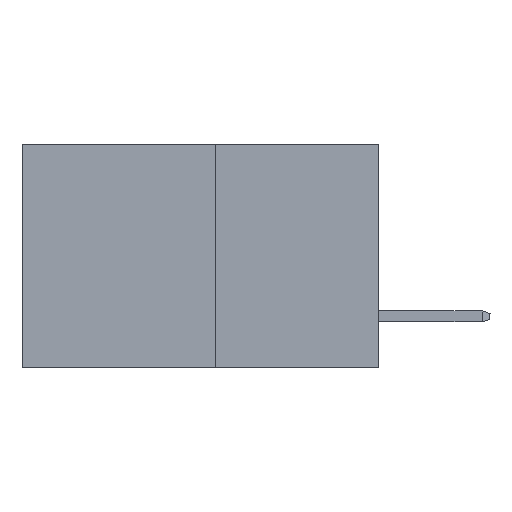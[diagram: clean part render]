
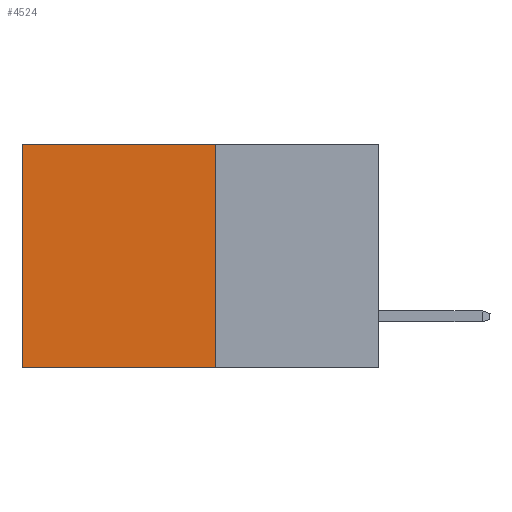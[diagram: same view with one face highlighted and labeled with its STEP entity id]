
A CAD part, left-side view. The second image highlights one B-rep face of the part: STEP entity #4524.
In plain terms, the highlighted planar face has unit normal (-1, 0, 0).
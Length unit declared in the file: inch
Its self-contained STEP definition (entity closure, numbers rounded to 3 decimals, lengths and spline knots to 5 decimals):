
#132 = VECTOR ( 'NONE', #27790, 39.37008 ) ;
#869 = LINE ( 'NONE', #1344, #132 ) ;
#1261 = CARTESIAN_POINT ( 'NONE',  ( 0.277, 0.59, 0. ) ) ;
#1344 = CARTESIAN_POINT ( 'NONE',  ( 0.277, 0.27, -0.37 ) ) ;
#2692 = DIRECTION ( 'NONE',  ( 0., 0., -1. ) ) ;
#3535 = ORIENTED_EDGE ( 'NONE', *, *, #17975, .T. ) ;
#4341 = CARTESIAN_POINT ( 'NONE',  ( 0.277, 0.27, -0.37 ) ) ;
#4524 = ADVANCED_FACE ( 'NONE', ( #17333 ), #16282, .F. ) ;
#4941 = EDGE_CURVE ( 'NONE', #23599, #19851, #16591, .T. ) ;
#6849 = CARTESIAN_POINT ( 'NONE',  ( 0.277, 0.59, -0.37 ) ) ;
#7403 = VECTOR ( 'NONE', #23509, 39.37008 ) ;
#7440 = VERTEX_POINT ( 'NONE', #21478 ) ;
#8963 = CARTESIAN_POINT ( 'NONE',  ( 0.277, 0.27, -0.37 ) ) ;
#9587 = AXIS2_PLACEMENT_3D ( 'NONE', #17483, #15407, #20422 ) ;
#10596 = ORIENTED_EDGE ( 'NONE', *, *, #11051, .F. ) ;
#10961 = ORIENTED_EDGE ( 'NONE', *, *, #4941, .T. ) ;
#11051 = EDGE_CURVE ( 'NONE', #14256, #19851, #869, .T. ) ;
#13457 = CARTESIAN_POINT ( 'NONE',  ( 0.277, 0.59, -0.37 ) ) ;
#14256 = VERTEX_POINT ( 'NONE', #8963 ) ;
#14307 = CARTESIAN_POINT ( 'NONE',  ( 0.277, 0.27, 0. ) ) ;
#15407 = DIRECTION ( 'NONE',  ( 1., 0., 0. ) ) ;
#16282 = PLANE ( 'NONE',  #9587 ) ;
#16591 = LINE ( 'NONE', #13457, #28057 ) ;
#17333 = FACE_OUTER_BOUND ( 'NONE', #25717, .T. ) ;
#17483 = CARTESIAN_POINT ( 'NONE',  ( 0.277, 0.27, -0.37 ) ) ;
#17626 = VECTOR ( 'NONE', #29599, 39.37008 ) ;
#17975 = EDGE_CURVE ( 'NONE', #7440, #23599, #25696, .T. ) ;
#19851 = VERTEX_POINT ( 'NONE', #6849 ) ;
#20422 = DIRECTION ( 'NONE',  ( 0., 0., -1. ) ) ;
#21478 = CARTESIAN_POINT ( 'NONE',  ( 0.277, 0.27, 0. ) ) ;
#23509 = DIRECTION ( 'NONE',  ( 0., 1., 0. ) ) ;
#23599 = VERTEX_POINT ( 'NONE', #1261 ) ;
#24480 = LINE ( 'NONE', #4341, #17626 ) ;
#25017 = ORIENTED_EDGE ( 'NONE', *, *, #28580, .F. ) ;
#25696 = LINE ( 'NONE', #14307, #7403 ) ;
#25717 = EDGE_LOOP ( 'NONE', ( #10961, #10596, #25017, #3535 ) ) ;
#27790 = DIRECTION ( 'NONE',  ( 0., 1., 0. ) ) ;
#28057 = VECTOR ( 'NONE', #2692, 39.37008 ) ;
#28580 = EDGE_CURVE ( 'NONE', #7440, #14256, #24480, .T. ) ;
#29599 = DIRECTION ( 'NONE',  ( 0., 0., -1. ) ) ;
